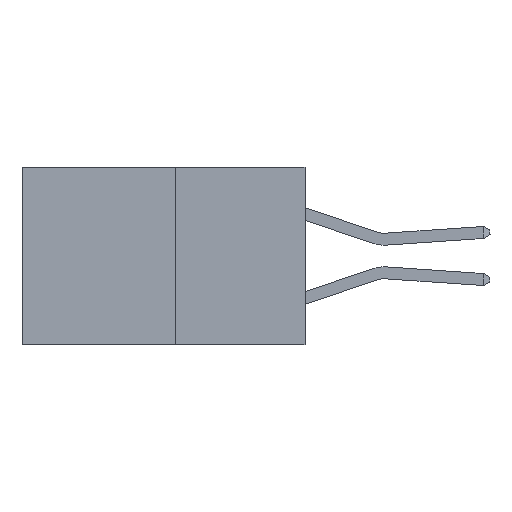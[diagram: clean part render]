
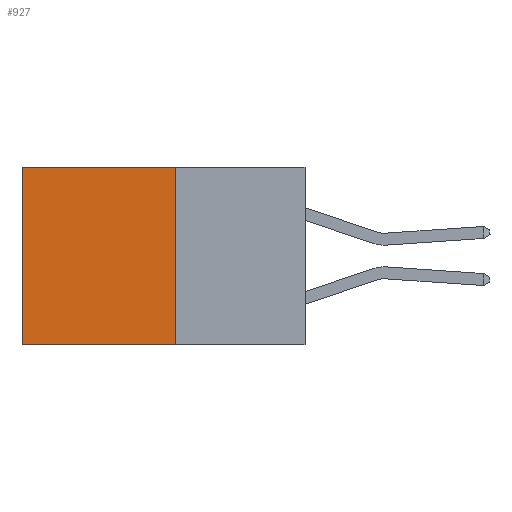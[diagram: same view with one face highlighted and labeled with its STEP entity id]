
A CAD part, left-side view. The second image highlights one B-rep face of the part: STEP entity #927.
In plain terms, the highlighted planar face has unit normal (-1, 0, 0).
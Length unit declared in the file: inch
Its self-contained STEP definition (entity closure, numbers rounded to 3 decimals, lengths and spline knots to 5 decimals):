
#799 = CARTESIAN_POINT ( 'NONE',  ( 0.277, 0.27, 0. ) ) ;
#927 = ADVANCED_FACE ( 'NONE', ( #8764 ), #12477, .F. ) ;
#1368 = VECTOR ( 'NONE', #12988, 39.37008 ) ;
#1498 = CARTESIAN_POINT ( 'NONE',  ( 0.277, 0.27, -0.37 ) ) ;
#1911 = VERTEX_POINT ( 'NONE', #5282 ) ;
#2691 = VERTEX_POINT ( 'NONE', #13298 ) ;
#3014 = ORIENTED_EDGE ( 'NONE', *, *, #16829, .F. ) ;
#4305 = CARTESIAN_POINT ( 'NONE',  ( 0.277, 0.27, 0. ) ) ;
#4365 = CARTESIAN_POINT ( 'NONE',  ( 0.277, 0.27, -0.37 ) ) ;
#4698 = VERTEX_POINT ( 'NONE', #4305 ) ;
#5282 = CARTESIAN_POINT ( 'NONE',  ( 0.277, 0.59, 0. ) ) ;
#6390 = DIRECTION ( 'NONE',  ( 0., 0., -1. ) ) ;
#6444 = ORIENTED_EDGE ( 'NONE', *, *, #17255, .T. ) ;
#6636 = AXIS2_PLACEMENT_3D ( 'NONE', #4365, #14769, #6771 ) ;
#6759 = VECTOR ( 'NONE', #6390, 39.37008 ) ;
#6771 = DIRECTION ( 'NONE',  ( 0., 0., -1. ) ) ;
#8029 = EDGE_CURVE ( 'NONE', #4698, #2691, #12654, .T. ) ;
#8385 = VECTOR ( 'NONE', #13614, 39.37008 ) ;
#8523 = VECTOR ( 'NONE', #11663, 39.37008 ) ;
#8673 = ORIENTED_EDGE ( 'NONE', *, *, #8029, .F. ) ;
#8764 = FACE_OUTER_BOUND ( 'NONE', #17217, .T. ) ;
#8808 = LINE ( 'NONE', #1498, #8385 ) ;
#8918 = ORIENTED_EDGE ( 'NONE', *, *, #12376, .T. ) ;
#8933 = CARTESIAN_POINT ( 'NONE',  ( 0.277, 0.59, -0.37 ) ) ;
#10202 = CARTESIAN_POINT ( 'NONE',  ( 0.277, 0.59, -0.37 ) ) ;
#10528 = VERTEX_POINT ( 'NONE', #10202 ) ;
#11663 = DIRECTION ( 'NONE',  ( 0., 1., 0. ) ) ;
#12376 = EDGE_CURVE ( 'NONE', #4698, #1911, #15990, .T. ) ;
#12477 = PLANE ( 'NONE',  #6636 ) ;
#12654 = LINE ( 'NONE', #14428, #6759 ) ;
#12988 = DIRECTION ( 'NONE',  ( 0., 0., -1. ) ) ;
#13298 = CARTESIAN_POINT ( 'NONE',  ( 0.277, 0.27, -0.37 ) ) ;
#13614 = DIRECTION ( 'NONE',  ( 0., 1., 0. ) ) ;
#14428 = CARTESIAN_POINT ( 'NONE',  ( 0.277, 0.27, -0.37 ) ) ;
#14769 = DIRECTION ( 'NONE',  ( 1., 0., 0. ) ) ;
#15671 = LINE ( 'NONE', #8933, #1368 ) ;
#15990 = LINE ( 'NONE', #799, #8523 ) ;
#16829 = EDGE_CURVE ( 'NONE', #2691, #10528, #8808, .T. ) ;
#17217 = EDGE_LOOP ( 'NONE', ( #6444, #3014, #8673, #8918 ) ) ;
#17255 = EDGE_CURVE ( 'NONE', #1911, #10528, #15671, .T. ) ;
